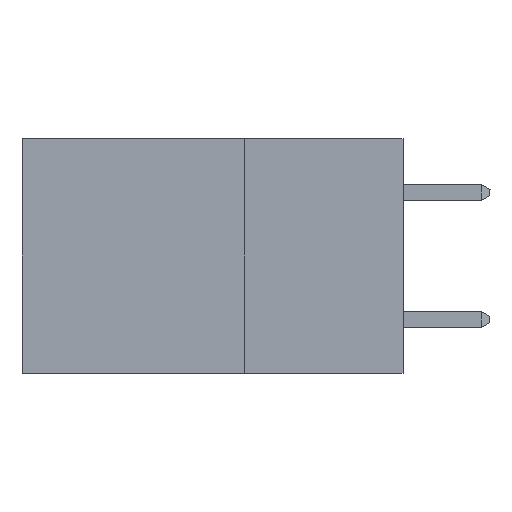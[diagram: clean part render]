
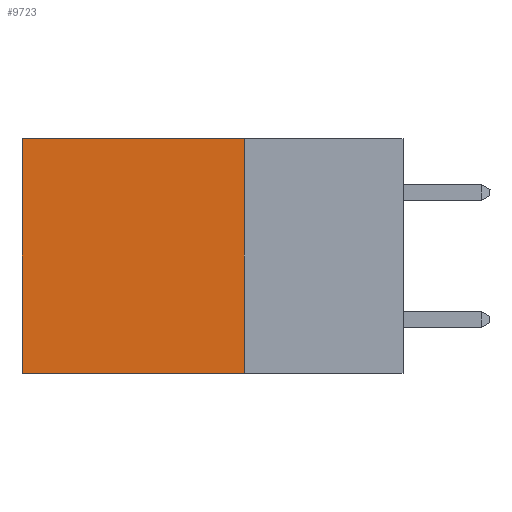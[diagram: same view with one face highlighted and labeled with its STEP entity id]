
A CAD part, left-side view. The second image highlights one B-rep face of the part: STEP entity #9723.
In plain terms, the highlighted planar face has unit normal (-1, 0, 0).
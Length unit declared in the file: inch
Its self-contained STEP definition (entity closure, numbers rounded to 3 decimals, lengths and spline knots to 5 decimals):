
#74 = ORIENTED_EDGE ( 'NONE', *, *, #12407, .F. ) ;
#679 = CARTESIAN_POINT ( 'NONE',  ( 0.2875, 0.6, 0. ) ) ;
#3236 = EDGE_CURVE ( 'NONE', #8928, #20639, #21739, .T. ) ;
#3517 = DIRECTION ( 'NONE',  ( 0., 0., -1. ) ) ;
#3957 = EDGE_LOOP ( 'NONE', ( #4431, #74, #18801, #11015 ) ) ;
#4431 = ORIENTED_EDGE ( 'NONE', *, *, #3236, .T. ) ;
#5018 = VERTEX_POINT ( 'NONE', #13012 ) ;
#5949 = LINE ( 'NONE', #7495, #9968 ) ;
#6428 = CARTESIAN_POINT ( 'NONE',  ( 0.2875, 0.25, -0.37 ) ) ;
#7440 = PLANE ( 'NONE',  #14792 ) ;
#7495 = CARTESIAN_POINT ( 'NONE',  ( 0.2875, 0.25, 0. ) ) ;
#8696 = CARTESIAN_POINT ( 'NONE',  ( 0.2875, 0.25, 0. ) ) ;
#8928 = VERTEX_POINT ( 'NONE', #679 ) ;
#9479 = DIRECTION ( 'NONE',  ( 0., 0., -1. ) ) ;
#9723 = ADVANCED_FACE ( 'NONE', ( #16232 ), #7440, .F. ) ;
#9968 = VECTOR ( 'NONE', #9479, 39.37008 ) ;
#10215 = CARTESIAN_POINT ( 'NONE',  ( 0.2875, 0.25, -0.37 ) ) ;
#10433 = EDGE_CURVE ( 'NONE', #5018, #16034, #5949, .T. ) ;
#11015 = ORIENTED_EDGE ( 'NONE', *, *, #13255, .T. ) ;
#11396 = VECTOR ( 'NONE', #24016, 39.37008 ) ;
#11401 = DIRECTION ( 'NONE',  ( 1., 0., 0. ) ) ;
#12177 = CARTESIAN_POINT ( 'NONE',  ( 0.2875, 0.6, -0.37 ) ) ;
#12407 = EDGE_CURVE ( 'NONE', #16034, #20639, #16085, .T. ) ;
#12599 = LINE ( 'NONE', #8696, #17876 ) ;
#13012 = CARTESIAN_POINT ( 'NONE',  ( 0.2875, 0.25, 0. ) ) ;
#13255 = EDGE_CURVE ( 'NONE', #5018, #8928, #12599, .T. ) ;
#14792 = AXIS2_PLACEMENT_3D ( 'NONE', #23238, #11401, #25189 ) ;
#15419 = CARTESIAN_POINT ( 'NONE',  ( 0.2875, 0.6, 0. ) ) ;
#16034 = VERTEX_POINT ( 'NONE', #6428 ) ;
#16085 = LINE ( 'NONE', #10215, #11396 ) ;
#16232 = FACE_OUTER_BOUND ( 'NONE', #3957, .T. ) ;
#17876 = VECTOR ( 'NONE', #22528, 39.37008 ) ;
#18801 = ORIENTED_EDGE ( 'NONE', *, *, #10433, .F. ) ;
#20639 = VERTEX_POINT ( 'NONE', #12177 ) ;
#21739 = LINE ( 'NONE', #15419, #25705 ) ;
#22528 = DIRECTION ( 'NONE',  ( 0., 1., 0. ) ) ;
#23238 = CARTESIAN_POINT ( 'NONE',  ( 0.2875, 0.25, 0. ) ) ;
#24016 = DIRECTION ( 'NONE',  ( 0., 1., 0. ) ) ;
#25189 = DIRECTION ( 'NONE',  ( 0., 0., -1. ) ) ;
#25705 = VECTOR ( 'NONE', #3517, 39.37008 ) ;
